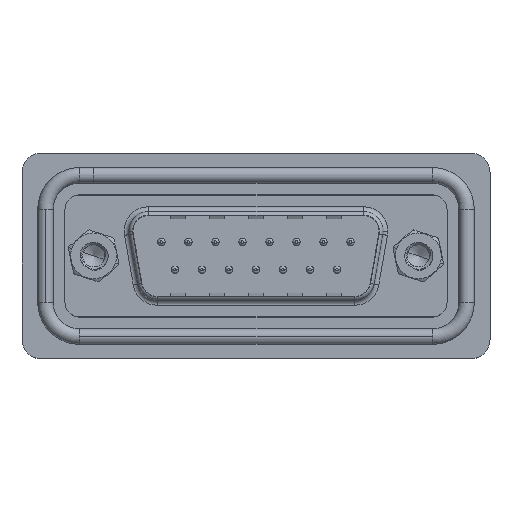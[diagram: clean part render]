
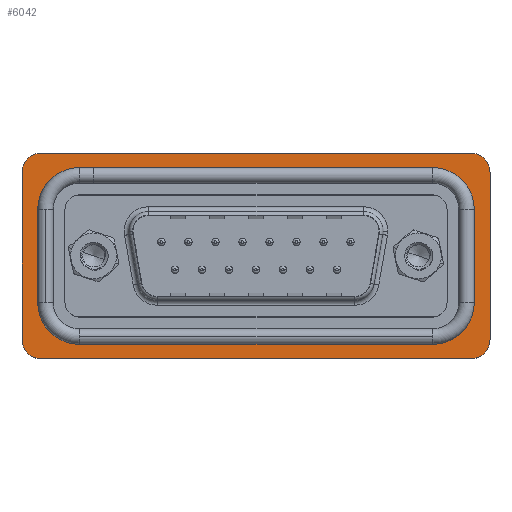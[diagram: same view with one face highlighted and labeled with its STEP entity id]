
A CAD part, top view. The second image highlights one B-rep face of the part: STEP entity #6042.
In plain terms, the highlighted planar face has unit normal (0, 0, 1).
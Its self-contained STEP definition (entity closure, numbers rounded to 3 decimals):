
#1 = DIRECTION ( 'NONE',  ( 1., 0., 0. ) ) ;
#144 = DIRECTION ( 'NONE',  ( 0., 0., 1. ) ) ;
#548 = CARTESIAN_POINT ( 'NONE',  ( -5.745, 4.775, 0.5 ) ) ;
#574 = VERTEX_POINT ( 'NONE', #4272 ) ;
#675 = VERTEX_POINT ( 'NONE', #23136 ) ;
#723 = CARTESIAN_POINT ( 'NONE',  ( -1.445, -4.775, 0.5 ) ) ;
#851 = EDGE_CURVE ( 'NONE', #675, #5980, #16521, .T. ) ;
#870 = EDGE_CURVE ( 'NONE', #10728, #18896, #9455, .T. ) ;
#1042 = CIRCLE ( 'NONE', #21772, 4.3 ) ;
#1119 = DIRECTION ( 'NONE',  ( 0., 1., 0. ) ) ;
#1231 = EDGE_CURVE ( 'NONE', #18782, #4588, #1042, .T. ) ;
#2167 = AXIS2_PLACEMENT_3D ( 'NONE', #17906, #16360, #19784 ) ;
#2419 = VERTEX_POINT ( 'NONE', #10241 ) ;
#2439 = EDGE_CURVE ( 'NONE', #2419, #18794, #4835, .T. ) ;
#2691 = ORIENTED_EDGE ( 'NONE', *, *, #21393, .F. ) ;
#2757 = DIRECTION ( 'NONE',  ( -1., 0., 0. ) ) ;
#2771 = ORIENTED_EDGE ( 'NONE', *, *, #1231, .F. ) ;
#2918 = CIRCLE ( 'NONE', #2167, 2. ) ;
#3143 = CARTESIAN_POINT ( 'NONE',  ( 39.045, -4.775, 0.5 ) ) ;
#3161 = DIRECTION ( 'NONE',  ( 0., 0., 1. ) ) ;
#3282 = VECTOR ( 'NONE', #1, 1000. ) ;
#3329 = VECTOR ( 'NONE', #21056, 1000. ) ;
#3696 = AXIS2_PLACEMENT_3D ( 'NONE', #6301, #20702, #4542 ) ;
#3798 = CARTESIAN_POINT ( 'NONE',  ( 34.745, 9.075, 0.5 ) ) ;
#4014 = CARTESIAN_POINT ( 'NONE',  ( -1.445, 9.075, 0.5 ) ) ;
#4272 = CARTESIAN_POINT ( 'NONE',  ( 38.65, 10.55, 0.5 ) ) ;
#4430 = AXIS2_PLACEMENT_3D ( 'NONE', #18555, #13607, #7930 ) ;
#4542 = DIRECTION ( 'NONE',  ( 1., 0., 0. ) ) ;
#4588 = VERTEX_POINT ( 'NONE', #3798 ) ;
#4708 = EDGE_CURVE ( 'NONE', #5980, #10728, #19872, .T. ) ;
#4782 = CIRCLE ( 'NONE', #20985, 2. ) ;
#4835 = LINE ( 'NONE', #22307, #23162 ) ;
#5149 = EDGE_CURVE ( 'NONE', #574, #11581, #14416, .T. ) ;
#5763 = VERTEX_POINT ( 'NONE', #548 ) ;
#5777 = ORIENTED_EDGE ( 'NONE', *, *, #6747, .F. ) ;
#5778 = CARTESIAN_POINT ( 'NONE',  ( -7.35, 8.55, 0.5 ) ) ;
#5883 = DIRECTION ( 'NONE',  ( 1., 0., 0. ) ) ;
#5884 = CARTESIAN_POINT ( 'NONE',  ( 38.65, -10.55, 0.5 ) ) ;
#5918 = ORIENTED_EDGE ( 'NONE', *, *, #4708, .T. ) ;
#5980 = VERTEX_POINT ( 'NONE', #15317 ) ;
#6042 = ADVANCED_FACE ( 'NONE', ( #12113, #17777 ), #21660, .T. ) ;
#6199 = AXIS2_PLACEMENT_3D ( 'NONE', #7343, #144, #5883 ) ;
#6297 = DIRECTION ( 'NONE',  ( 1., 0., 0. ) ) ;
#6301 = CARTESIAN_POINT ( 'NONE',  ( -1.445, 4.775, 0.5 ) ) ;
#6711 = DIRECTION ( 'NONE',  ( -1., 0., 0. ) ) ;
#6747 = EDGE_CURVE ( 'NONE', #18794, #13230, #9990, .T. ) ;
#7139 = DIRECTION ( 'NONE',  ( 0., 0., 1. ) ) ;
#7253 = EDGE_LOOP ( 'NONE', ( #18759, #16555, #21985, #9967, #16709, #10676, #5918, #8011 ) ) ;
#7343 = CARTESIAN_POINT ( 'NONE',  ( 34.745, -4.775, 0.5 ) ) ;
#7930 = DIRECTION ( 'NONE',  ( 1., 0., 0. ) ) ;
#7999 = CARTESIAN_POINT ( 'NONE',  ( 34.745, -9.075, 0.5 ) ) ;
#8011 = ORIENTED_EDGE ( 'NONE', *, *, #870, .T. ) ;
#8246 = AXIS2_PLACEMENT_3D ( 'NONE', #723, #20544, #22432 ) ;
#8318 = CARTESIAN_POINT ( 'NONE',  ( 39.045, -4.775, 0.5 ) ) ;
#8341 = CARTESIAN_POINT ( 'NONE',  ( -5.745, -4.775, 0.5 ) ) ;
#8921 = CARTESIAN_POINT ( 'NONE',  ( 40.65, -8.55, 0.5 ) ) ;
#9023 = VECTOR ( 'NONE', #22860, 1000. ) ;
#9159 = CARTESIAN_POINT ( 'NONE',  ( 38.65, 8.55, 0.5 ) ) ;
#9207 = AXIS2_PLACEMENT_3D ( 'NONE', #9159, #7139, #23313 ) ;
#9396 = CIRCLE ( 'NONE', #8246, 4.3 ) ;
#9455 = LINE ( 'NONE', #21838, #10833 ) ;
#9619 = EDGE_CURVE ( 'NONE', #18896, #574, #4782, .T. ) ;
#9967 = ORIENTED_EDGE ( 'NONE', *, *, #11232, .T. ) ;
#9990 = CIRCLE ( 'NONE', #6199, 4.3 ) ;
#10241 = CARTESIAN_POINT ( 'NONE',  ( -1.445, -9.075, 0.5 ) ) ;
#10278 = DIRECTION ( 'NONE',  ( 1., 0., 0. ) ) ;
#10292 = ORIENTED_EDGE ( 'NONE', *, *, #2439, .F. ) ;
#10327 = CARTESIAN_POINT ( 'NONE',  ( -7.35, -8.55, 0.5 ) ) ;
#10676 = ORIENTED_EDGE ( 'NONE', *, *, #851, .T. ) ;
#10728 = VERTEX_POINT ( 'NONE', #8921 ) ;
#10833 = VECTOR ( 'NONE', #14419, 1000. ) ;
#11163 = EDGE_CURVE ( 'NONE', #17077, #5763, #16155, .T. ) ;
#11173 = EDGE_CURVE ( 'NONE', #19382, #675, #22553, .T. ) ;
#11232 = EDGE_CURVE ( 'NONE', #16424, #19382, #14221, .T. ) ;
#11581 = VERTEX_POINT ( 'NONE', #20875 ) ;
#11746 = CARTESIAN_POINT ( 'NONE',  ( -5.35, -8.55, 0.5 ) ) ;
#11811 = CARTESIAN_POINT ( 'NONE',  ( 34.745, 9.075, 0.5 ) ) ;
#11989 = LINE ( 'NONE', #8318, #16513 ) ;
#12067 = ORIENTED_EDGE ( 'NONE', *, *, #16621, .F. ) ;
#12113 = FACE_BOUND ( 'NONE', #16719, .T. ) ;
#12138 = ORIENTED_EDGE ( 'NONE', *, *, #11163, .F. ) ;
#12155 = LINE ( 'NONE', #11811, #19233 ) ;
#12379 = CARTESIAN_POINT ( 'NONE',  ( 34.745, 4.775, 0.5 ) ) ;
#12387 = AXIS2_PLACEMENT_3D ( 'NONE', #11746, #18933, #2757 ) ;
#12634 = DIRECTION ( 'NONE',  ( -1., 0., 0. ) ) ;
#13230 = VERTEX_POINT ( 'NONE', #3143 ) ;
#13422 = EDGE_CURVE ( 'NONE', #11581, #16424, #2918, .T. ) ;
#13607 = DIRECTION ( 'NONE',  ( 0., 0., 1. ) ) ;
#13833 = EDGE_CURVE ( 'NONE', #13230, #18782, #11989, .T. ) ;
#14221 = LINE ( 'NONE', #10327, #3329 ) ;
#14416 = LINE ( 'NONE', #21595, #21994 ) ;
#14419 = DIRECTION ( 'NONE',  ( 0., 1., 0. ) ) ;
#15293 = DIRECTION ( 'NONE',  ( 0., 0., 1. ) ) ;
#15317 = CARTESIAN_POINT ( 'NONE',  ( 38.65, -10.55, 0.5 ) ) ;
#15560 = LINE ( 'NONE', #22746, #9023 ) ;
#16018 = CARTESIAN_POINT ( 'NONE',  ( 40.65, 8.55, 0.5 ) ) ;
#16155 = CIRCLE ( 'NONE', #3696, 4.3 ) ;
#16360 = DIRECTION ( 'NONE',  ( 0., 0., 1. ) ) ;
#16424 = VERTEX_POINT ( 'NONE', #5778 ) ;
#16513 = VECTOR ( 'NONE', #1119, 1000. ) ;
#16521 = LINE ( 'NONE', #5884, #3282 ) ;
#16555 = ORIENTED_EDGE ( 'NONE', *, *, #5149, .T. ) ;
#16621 = EDGE_CURVE ( 'NONE', #4588, #17077, #12155, .T. ) ;
#16667 = ORIENTED_EDGE ( 'NONE', *, *, #13833, .F. ) ;
#16709 = ORIENTED_EDGE ( 'NONE', *, *, #11173, .T. ) ;
#16719 = EDGE_LOOP ( 'NONE', ( #2771, #16667, #5777, #10292, #23336, #2691, #12138, #12067 ) ) ;
#17077 = VERTEX_POINT ( 'NONE', #4014 ) ;
#17450 = DIRECTION ( 'NONE',  ( 1., 0., 0. ) ) ;
#17777 = FACE_OUTER_BOUND ( 'NONE', #7253, .T. ) ;
#17906 = CARTESIAN_POINT ( 'NONE',  ( -5.35, 8.55, 0.5 ) ) ;
#18555 = CARTESIAN_POINT ( 'NONE',  ( 38.65, -8.55, 0.5 ) ) ;
#18759 = ORIENTED_EDGE ( 'NONE', *, *, #9619, .T. ) ;
#18782 = VERTEX_POINT ( 'NONE', #22505 ) ;
#18794 = VERTEX_POINT ( 'NONE', #7999 ) ;
#18811 = VERTEX_POINT ( 'NONE', #8341 ) ;
#18896 = VERTEX_POINT ( 'NONE', #16018 ) ;
#18933 = DIRECTION ( 'NONE',  ( 0., 0., 1. ) ) ;
#19036 = CARTESIAN_POINT ( 'NONE',  ( 38.65, 8.55, 0.5 ) ) ;
#19233 = VECTOR ( 'NONE', #6711, 1000. ) ;
#19382 = VERTEX_POINT ( 'NONE', #21295 ) ;
#19784 = DIRECTION ( 'NONE',  ( 1., 0., 0. ) ) ;
#19872 = CIRCLE ( 'NONE', #4430, 2. ) ;
#20544 = DIRECTION ( 'NONE',  ( 0., 0., 1. ) ) ;
#20702 = DIRECTION ( 'NONE',  ( 0., 0., 1. ) ) ;
#20748 = EDGE_CURVE ( 'NONE', #18811, #2419, #9396, .T. ) ;
#20875 = CARTESIAN_POINT ( 'NONE',  ( -5.35, 10.55, 0.5 ) ) ;
#20985 = AXIS2_PLACEMENT_3D ( 'NONE', #19036, #15293, #6297 ) ;
#21056 = DIRECTION ( 'NONE',  ( 0., -1., 0. ) ) ;
#21295 = CARTESIAN_POINT ( 'NONE',  ( -7.35, -8.55, 0.5 ) ) ;
#21393 = EDGE_CURVE ( 'NONE', #5763, #18811, #15560, .T. ) ;
#21595 = CARTESIAN_POINT ( 'NONE',  ( 38.65, 10.55, 0.5 ) ) ;
#21660 = PLANE ( 'NONE',  #9207 ) ;
#21772 = AXIS2_PLACEMENT_3D ( 'NONE', #12379, #3161, #17450 ) ;
#21838 = CARTESIAN_POINT ( 'NONE',  ( 40.65, -8.55, 0.5 ) ) ;
#21985 = ORIENTED_EDGE ( 'NONE', *, *, #13422, .T. ) ;
#21994 = VECTOR ( 'NONE', #12634, 1000. ) ;
#22307 = CARTESIAN_POINT ( 'NONE',  ( -1.445, -9.075, 0.5 ) ) ;
#22432 = DIRECTION ( 'NONE',  ( 1., 0., 0. ) ) ;
#22505 = CARTESIAN_POINT ( 'NONE',  ( 39.045, 4.775, 0.5 ) ) ;
#22553 = CIRCLE ( 'NONE', #12387, 2. ) ;
#22746 = CARTESIAN_POINT ( 'NONE',  ( -5.745, 4.775, 0.5 ) ) ;
#22860 = DIRECTION ( 'NONE',  ( 0., -1., 0. ) ) ;
#23136 = CARTESIAN_POINT ( 'NONE',  ( -5.35, -10.55, 0.5 ) ) ;
#23162 = VECTOR ( 'NONE', #10278, 1000. ) ;
#23313 = DIRECTION ( 'NONE',  ( 1., 0., 0. ) ) ;
#23336 = ORIENTED_EDGE ( 'NONE', *, *, #20748, .F. ) ;
